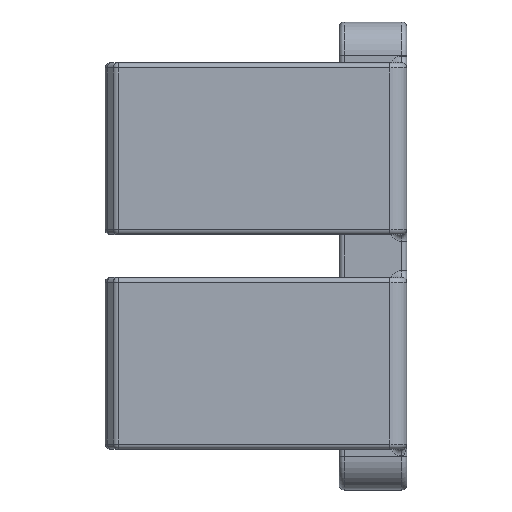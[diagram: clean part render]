
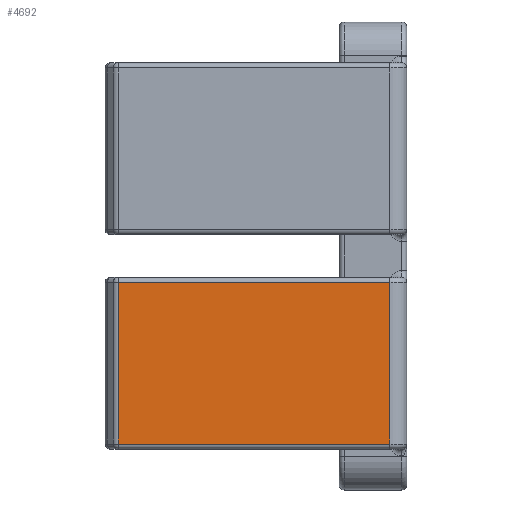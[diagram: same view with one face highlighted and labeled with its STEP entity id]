
A CAD part, left-side view. The second image highlights one B-rep face of the part: STEP entity #4692.
In plain terms, the highlighted planar face has unit normal (-1, 0, 0).
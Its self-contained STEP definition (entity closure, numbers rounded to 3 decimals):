
#229 = LINE ( 'NONE', #1902, #2584 ) ;
#284 = ORIENTED_EDGE ( 'NONE', *, *, #1834, .T. ) ;
#304 = LINE ( 'NONE', #3419, #3524 ) ;
#396 = CARTESIAN_POINT ( 'NONE',  ( -18.312, 48.07, 0. ) ) ;
#585 = VERTEX_POINT ( 'NONE', #913 ) ;
#658 = AXIS2_PLACEMENT_3D ( 'NONE', #3638, #1980, #4946 ) ;
#712 = ORIENTED_EDGE ( 'NONE', *, *, #4616, .T. ) ;
#906 = FACE_OUTER_BOUND ( 'NONE', #2068, .T. ) ;
#913 = CARTESIAN_POINT ( 'NONE',  ( -18.312, 7.884, -3.925 ) ) ;
#1033 = EDGE_CURVE ( 'NONE', #2935, #585, #5464, .T. ) ;
#1353 = ORIENTED_EDGE ( 'NONE', *, *, #3388, .T. ) ;
#1834 = EDGE_CURVE ( 'NONE', #585, #2690, #229, .T. ) ;
#1902 = CARTESIAN_POINT ( 'NONE',  ( -18.312, 48.07, -3.925 ) ) ;
#1980 = DIRECTION ( 'NONE',  ( -1., 0., 0. ) ) ;
#2068 = EDGE_LOOP ( 'NONE', ( #1353, #712, #5478, #284 ) ) ;
#2116 = LINE ( 'NONE', #396, #3099 ) ;
#2372 = PLANE ( 'NONE',  #658 ) ;
#2536 = VERTEX_POINT ( 'NONE', #4970 ) ;
#2584 = VECTOR ( 'NONE', #4426, 1000. ) ;
#2690 = VERTEX_POINT ( 'NONE', #4663 ) ;
#2935 = VERTEX_POINT ( 'NONE', #4764 ) ;
#3099 = VECTOR ( 'NONE', #3739, 1000. ) ;
#3388 = EDGE_CURVE ( 'NONE', #2690, #2536, #2116, .T. ) ;
#3419 = CARTESIAN_POINT ( 'NONE',  ( -18.312, 7.884, -27.825 ) ) ;
#3524 = VECTOR ( 'NONE', #4704, 1000. ) ;
#3576 = DIRECTION ( 'NONE',  ( 0., 0., 1. ) ) ;
#3638 = CARTESIAN_POINT ( 'NONE',  ( -18.312, 0., 0. ) ) ;
#3739 = DIRECTION ( 'NONE',  ( 0., 0., -1. ) ) ;
#4002 = CARTESIAN_POINT ( 'NONE',  ( -18.312, 7.884, -3.175 ) ) ;
#4317 = VECTOR ( 'NONE', #3576, 1000. ) ;
#4426 = DIRECTION ( 'NONE',  ( 0., 1., 0. ) ) ;
#4616 = EDGE_CURVE ( 'NONE', #2536, #2935, #304, .T. ) ;
#4663 = CARTESIAN_POINT ( 'NONE',  ( -18.312, 48.07, -3.925 ) ) ;
#4692 = ADVANCED_FACE ( 'NONE', ( #906 ), #2372, .T. ) ;
#4704 = DIRECTION ( 'NONE',  ( 0., -1., 0. ) ) ;
#4764 = CARTESIAN_POINT ( 'NONE',  ( -18.312, 7.884, -27.825 ) ) ;
#4946 = DIRECTION ( 'NONE',  ( 0., 0., 1. ) ) ;
#4970 = CARTESIAN_POINT ( 'NONE',  ( -18.312, 48.07, -27.825 ) ) ;
#5464 = LINE ( 'NONE', #4002, #4317 ) ;
#5478 = ORIENTED_EDGE ( 'NONE', *, *, #1033, .T. ) ;
